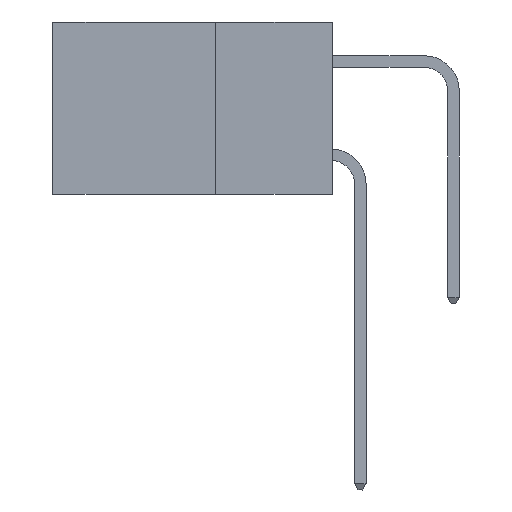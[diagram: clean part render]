
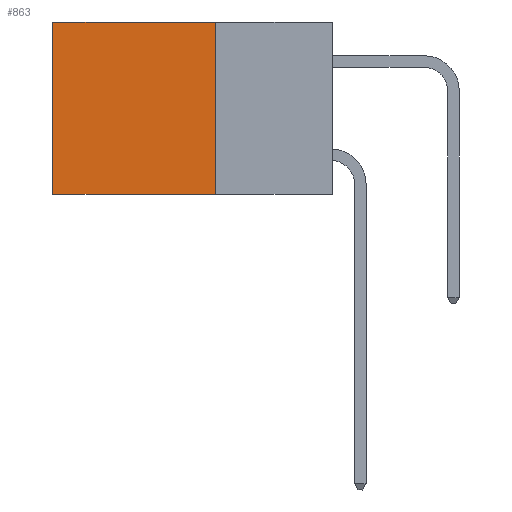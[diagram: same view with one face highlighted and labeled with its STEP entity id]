
A CAD part, left-side view. The second image highlights one B-rep face of the part: STEP entity #863.
In plain terms, the highlighted planar face has unit normal (-1, 0, 0).
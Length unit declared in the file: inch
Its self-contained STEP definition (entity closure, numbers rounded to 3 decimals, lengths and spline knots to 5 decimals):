
#449 = DIRECTION ( 'NONE',  ( 0., 1., 0. ) ) ;
#568 = CARTESIAN_POINT ( 'NONE',  ( 0.298, 0.25, 0. ) ) ;
#621 = VECTOR ( 'NONE', #9230, 39.37008 ) ;
#749 = DIRECTION ( 'NONE',  ( 0., 0., -1. ) ) ;
#863 = ADVANCED_FACE ( 'NONE', ( #8039 ), #12034, .F. ) ;
#1159 = CARTESIAN_POINT ( 'NONE',  ( 0.298, 0.6, 0. ) ) ;
#1327 = VECTOR ( 'NONE', #449, 39.37008 ) ;
#1965 = ORIENTED_EDGE ( 'NONE', *, *, #12380, .F. ) ;
#2101 = DIRECTION ( 'NONE',  ( 0., 0., -1. ) ) ;
#2325 = VERTEX_POINT ( 'NONE', #1159 ) ;
#3055 = CARTESIAN_POINT ( 'NONE',  ( 0.298, 0.6, 0. ) ) ;
#4247 = EDGE_CURVE ( 'NONE', #6335, #12248, #6111, .T. ) ;
#4365 = CARTESIAN_POINT ( 'NONE',  ( 0.298, 0.25, 0. ) ) ;
#4972 = VERTEX_POINT ( 'NONE', #5677 ) ;
#5677 = CARTESIAN_POINT ( 'NONE',  ( 0.298, 0.6, -0.37 ) ) ;
#6111 = LINE ( 'NONE', #4365, #8691 ) ;
#6148 = ORIENTED_EDGE ( 'NONE', *, *, #7871, .T. ) ;
#6193 = CARTESIAN_POINT ( 'NONE',  ( 0.298, 0.25, 0. ) ) ;
#6335 = VERTEX_POINT ( 'NONE', #8362 ) ;
#6687 = LINE ( 'NONE', #11019, #1327 ) ;
#7649 = EDGE_LOOP ( 'NONE', ( #6148, #1965, #10206, #10060 ) ) ;
#7871 = EDGE_CURVE ( 'NONE', #2325, #4972, #8949, .T. ) ;
#8039 = FACE_OUTER_BOUND ( 'NONE', #7649, .T. ) ;
#8351 = DIRECTION ( 'NONE',  ( 0., 0., -1. ) ) ;
#8362 = CARTESIAN_POINT ( 'NONE',  ( 0.298, 0.25, 0. ) ) ;
#8593 = LINE ( 'NONE', #568, #621 ) ;
#8691 = VECTOR ( 'NONE', #8351, 39.37008 ) ;
#8949 = LINE ( 'NONE', #3055, #11173 ) ;
#9220 = AXIS2_PLACEMENT_3D ( 'NONE', #6193, #11100, #749 ) ;
#9230 = DIRECTION ( 'NONE',  ( 0., 1., 0. ) ) ;
#10060 = ORIENTED_EDGE ( 'NONE', *, *, #10437, .T. ) ;
#10206 = ORIENTED_EDGE ( 'NONE', *, *, #4247, .F. ) ;
#10437 = EDGE_CURVE ( 'NONE', #6335, #2325, #8593, .T. ) ;
#10813 = CARTESIAN_POINT ( 'NONE',  ( 0.298, 0.25, -0.37 ) ) ;
#11019 = CARTESIAN_POINT ( 'NONE',  ( 0.298, 0.25, -0.37 ) ) ;
#11100 = DIRECTION ( 'NONE',  ( 1., 0., 0. ) ) ;
#11173 = VECTOR ( 'NONE', #2101, 39.37008 ) ;
#12034 = PLANE ( 'NONE',  #9220 ) ;
#12248 = VERTEX_POINT ( 'NONE', #10813 ) ;
#12380 = EDGE_CURVE ( 'NONE', #12248, #4972, #6687, .T. ) ;
